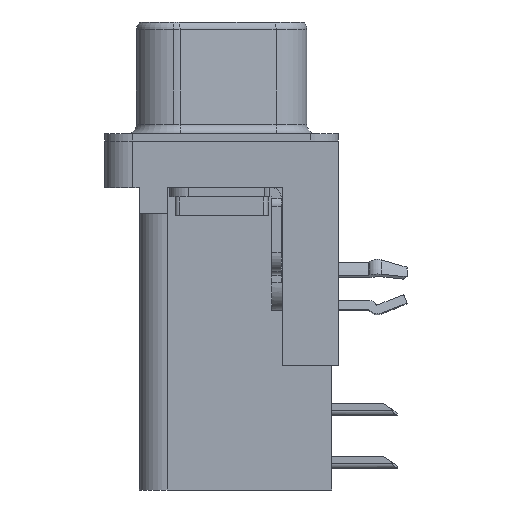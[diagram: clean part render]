
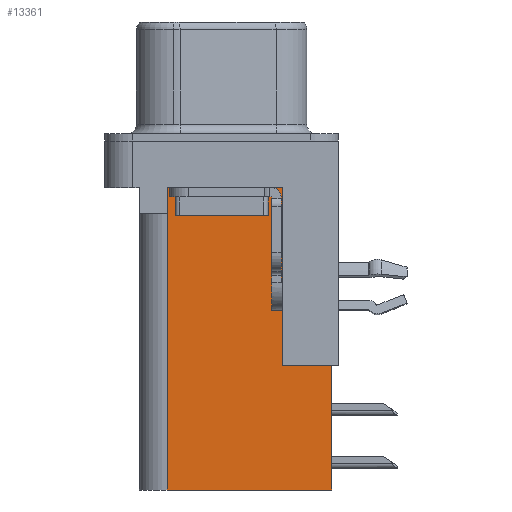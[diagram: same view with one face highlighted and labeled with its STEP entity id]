
A CAD part, left-side view. The second image highlights one B-rep face of the part: STEP entity #13361.
In plain terms, the highlighted planar face has unit normal (-1, 0, 0).
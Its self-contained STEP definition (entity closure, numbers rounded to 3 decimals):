
#214 = VERTEX_POINT ( 'NONE', #17296 ) ;
#441 = VERTEX_POINT ( 'NONE', #19008 ) ;
#558 = VERTEX_POINT ( 'NONE', #6761 ) ;
#1655 = EDGE_CURVE ( 'NONE', #7824, #4925, #16865, .T. ) ;
#1828 = VECTOR ( 'NONE', #8444, 1000. ) ;
#1969 = CARTESIAN_POINT ( 'NONE',  ( 3.765, -3.295, -2.5 ) ) ;
#2222 = CARTESIAN_POINT ( 'NONE',  ( 3.765, 2.895, -3.9 ) ) ;
#2527 = CARTESIAN_POINT ( 'NONE',  ( 3.765, -5.925, -2. ) ) ;
#2876 = EDGE_LOOP ( 'NONE', ( #8070, #8568, #8942, #17309, #16269, #3857, #4449, #2977 ) ) ;
#2977 = ORIENTED_EDGE ( 'NONE', *, *, #4079, .T. ) ;
#3290 = CARTESIAN_POINT ( 'NONE',  ( 3.765, -3.295, -18.76 ) ) ;
#3683 = EDGE_CURVE ( 'NONE', #441, #12416, #8874, .T. ) ;
#3857 = ORIENTED_EDGE ( 'NONE', *, *, #3683, .F. ) ;
#3887 = VECTOR ( 'NONE', #5704, 1000. ) ;
#3955 = EDGE_CURVE ( 'NONE', #12416, #7824, #7872, .T. ) ;
#4046 = LINE ( 'NONE', #4089, #3887 ) ;
#4079 = EDGE_CURVE ( 'NONE', #14396, #214, #7411, .T. ) ;
#4089 = CARTESIAN_POINT ( 'NONE',  ( 3.765, 0., -3.9 ) ) ;
#4268 = EDGE_CURVE ( 'NONE', #441, #14396, #6453, .T. ) ;
#4449 = ORIENTED_EDGE ( 'NONE', *, *, #4268, .T. ) ;
#4857 = VERTEX_POINT ( 'NONE', #2222 ) ;
#4925 = VERTEX_POINT ( 'NONE', #7058 ) ;
#4932 = PLANE ( 'NONE',  #16322 ) ;
#5521 = DIRECTION ( 'NONE',  ( 0., 0., -1. ) ) ;
#5704 = DIRECTION ( 'NONE',  ( 0., 1., 0. ) ) ;
#6453 = LINE ( 'NONE', #9305, #6540 ) ;
#6513 = DIRECTION ( 'NONE',  ( 0., 1., 0. ) ) ;
#6540 = VECTOR ( 'NONE', #6580, 1000. ) ;
#6580 = DIRECTION ( 'NONE',  ( 0., 1., 0. ) ) ;
#6761 = CARTESIAN_POINT ( 'NONE',  ( 3.765, 2.895, -2.5 ) ) ;
#7058 = CARTESIAN_POINT ( 'NONE',  ( 3.765, 2.925, -3.9 ) ) ;
#7287 = VECTOR ( 'NONE', #18647, 1000. ) ;
#7411 = LINE ( 'NONE', #18487, #7287 ) ;
#7483 = CARTESIAN_POINT ( 'NONE',  ( 3.765, -3.295, -18.76 ) ) ;
#7824 = VERTEX_POINT ( 'NONE', #14223 ) ;
#7854 = VECTOR ( 'NONE', #10489, 1000. ) ;
#7872 = LINE ( 'NONE', #7483, #7854 ) ;
#8070 = ORIENTED_EDGE ( 'NONE', *, *, #12714, .T. ) ;
#8444 = DIRECTION ( 'NONE',  ( 0., 1., 0. ) ) ;
#8568 = ORIENTED_EDGE ( 'NONE', *, *, #18868, .T. ) ;
#8840 = VECTOR ( 'NONE', #19076, 1000. ) ;
#8874 = LINE ( 'NONE', #2527, #8840 ) ;
#8942 = ORIENTED_EDGE ( 'NONE', *, *, #20443, .T. ) ;
#9305 = CARTESIAN_POINT ( 'NONE',  ( 3.765, -6.295, -12.05 ) ) ;
#10357 = CARTESIAN_POINT ( 'NONE',  ( 3.765, -3.295, -12.05 ) ) ;
#10489 = DIRECTION ( 'NONE',  ( 0., 1., 0. ) ) ;
#11384 = LINE ( 'NONE', #1969, #1828 ) ;
#12159 = FACE_OUTER_BOUND ( 'NONE', #2876, .T. ) ;
#12416 = VERTEX_POINT ( 'NONE', #17189 ) ;
#12697 = VECTOR ( 'NONE', #5521, 1000. ) ;
#12714 = EDGE_CURVE ( 'NONE', #214, #558, #11384, .T. ) ;
#12789 = LINE ( 'NONE', #13541, #12697 ) ;
#12879 = DIRECTION ( 'NONE',  ( 1., 0., 0. ) ) ;
#13361 = ADVANCED_FACE ( 'NONE', ( #12159 ), #4932, .F. ) ;
#13541 = CARTESIAN_POINT ( 'NONE',  ( 3.765, 2.895, -3.9 ) ) ;
#14223 = CARTESIAN_POINT ( 'NONE',  ( 3.765, 2.925, -18.76 ) ) ;
#14396 = VERTEX_POINT ( 'NONE', #10357 ) ;
#16269 = ORIENTED_EDGE ( 'NONE', *, *, #3955, .F. ) ;
#16322 = AXIS2_PLACEMENT_3D ( 'NONE', #3290, #12879, #6513 ) ;
#16787 = VECTOR ( 'NONE', #18086, 1000. ) ;
#16865 = LINE ( 'NONE', #20100, #16787 ) ;
#17189 = CARTESIAN_POINT ( 'NONE',  ( 3.765, -5.925, -18.76 ) ) ;
#17296 = CARTESIAN_POINT ( 'NONE',  ( 3.765, -3.295, -2.5 ) ) ;
#17309 = ORIENTED_EDGE ( 'NONE', *, *, #1655, .F. ) ;
#18086 = DIRECTION ( 'NONE',  ( 0., 0., 1. ) ) ;
#18487 = CARTESIAN_POINT ( 'NONE',  ( 3.765, -3.295, -18.76 ) ) ;
#18647 = DIRECTION ( 'NONE',  ( 0., 0., 1. ) ) ;
#18868 = EDGE_CURVE ( 'NONE', #558, #4857, #12789, .T. ) ;
#19008 = CARTESIAN_POINT ( 'NONE',  ( 3.765, -5.925, -12.05 ) ) ;
#19076 = DIRECTION ( 'NONE',  ( 0., 0., -1. ) ) ;
#20100 = CARTESIAN_POINT ( 'NONE',  ( 3.765, 2.925, -18.76 ) ) ;
#20443 = EDGE_CURVE ( 'NONE', #4857, #4925, #4046, .T. ) ;
